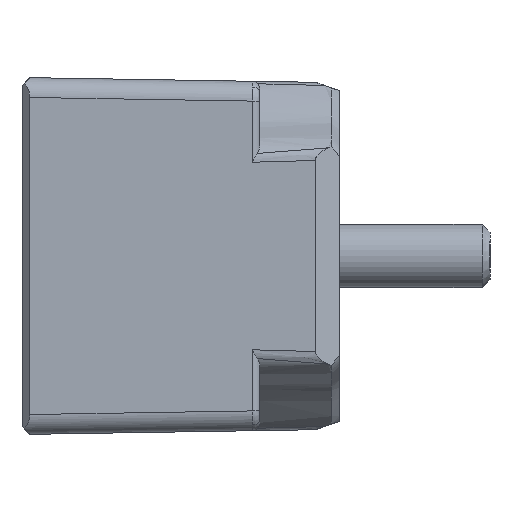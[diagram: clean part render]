
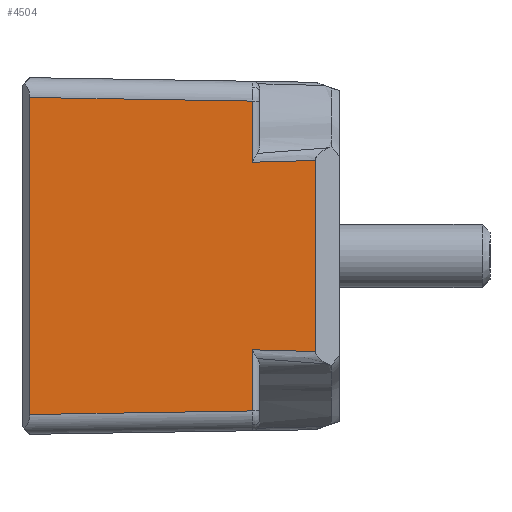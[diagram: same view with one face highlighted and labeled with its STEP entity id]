
A CAD part, left-side view. The second image highlights one B-rep face of the part: STEP entity #4504.
In plain terms, the highlighted planar face has unit normal (-1, -0.016, 0).
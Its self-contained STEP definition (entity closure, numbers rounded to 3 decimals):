
#189 = DIRECTION ( 'NONE',  ( -0.016, 1., 0.016 ) ) ;
#401 = CARTESIAN_POINT ( 'NONE',  ( -8.493, -0.1, -1.998 ) ) ;
#539 = CARTESIAN_POINT ( 'NONE',  ( -8.441, -3.302, -1.195 ) ) ;
#622 = CARTESIAN_POINT ( 'NONE',  ( -8.448, -2.902, 1.182 ) ) ;
#647 = CARTESIAN_POINT ( 'NONE',  ( -8.448, -2.902, -1.182 ) ) ;
#701 = CARTESIAN_POINT ( 'NONE',  ( -8.444, -3.169, -1.191 ) ) ;
#886 = ORIENTED_EDGE ( 'NONE', *, *, #1917, .T. ) ;
#990 = EDGE_CURVE ( 'NONE', #6883, #4766, #9644, .T. ) ;
#1015 = CARTESIAN_POINT ( 'NONE',  ( -8.448, -2.902, -1.182 ) ) ;
#1017 = VECTOR ( 'NONE', #8987, 1000. ) ;
#1172 = VECTOR ( 'NONE', #3954, 1000. ) ;
#1199 = EDGE_CURVE ( 'NONE', #4766, #1500, #3119, .T. ) ;
#1486 = EDGE_CURVE ( 'NONE', #8436, #5840, #6258, .T. ) ;
#1500 = VERTEX_POINT ( 'NONE', #4595 ) ;
#1817 = CARTESIAN_POINT ( 'NONE',  ( -8.435, -3.7, -1.204 ) ) ;
#1917 = EDGE_CURVE ( 'NONE', #3069, #4911, #2349, .T. ) ;
#2194 = VERTEX_POINT ( 'NONE', #622 ) ;
#2322 = VECTOR ( 'NONE', #7334, 1000. ) ;
#2349 = LINE ( 'NONE', #9001, #1172 ) ;
#2478 = EDGE_LOOP ( 'NONE', ( #2952, #8226, #8989, #6694, #8135, #886, #8292, #9587 ) ) ;
#2861 = DIRECTION ( 'NONE',  ( -1., -0.016, 0. ) ) ;
#2952 = ORIENTED_EDGE ( 'NONE', *, *, #1199, .T. ) ;
#3061 = CARTESIAN_POINT ( 'NONE',  ( -8.435, -3.7, 2.185 ) ) ;
#3069 = VERTEX_POINT ( 'NONE', #401 ) ;
#3119 = LINE ( 'NONE', #3061, #1017 ) ;
#3138 = CARTESIAN_POINT ( 'NONE',  ( -8.448, -2.902, -2.25 ) ) ;
#3382 = CARTESIAN_POINT ( 'NONE',  ( -8.441, -3.302, 1.195 ) ) ;
#3643 = CARTESIAN_POINT ( 'NONE',  ( -8.448, -2.902, -1.953 ) ) ;
#3954 = DIRECTION ( 'NONE',  ( 0.016, -1., 0.016 ) ) ;
#3985 = EDGE_CURVE ( 'NONE', #2194, #8436, #4789, .T. ) ;
#4006 = CARTESIAN_POINT ( 'NONE',  ( -8.435, -3.7, -1.204 ) ) ;
#4289 = LINE ( 'NONE', #6779, #5571 ) ;
#4504 = ADVANCED_FACE ( 'NONE', ( #8359 ), #9360, .T. ) ;
#4595 = CARTESIAN_POINT ( 'NONE',  ( -8.435, -3.7, 1.204 ) ) ;
#4607 = EDGE_CURVE ( 'NONE', #4911, #6883, #8063, .T. ) ;
#4766 = VERTEX_POINT ( 'NONE', #1817 ) ;
#4789 = LINE ( 'NONE', #6610, #2322 ) ;
#4911 = VERTEX_POINT ( 'NONE', #3643 ) ;
#4972 = CARTESIAN_POINT ( 'NONE',  ( -8.448, -2.902, 1.953 ) ) ;
#4981 = CARTESIAN_POINT ( 'NONE',  ( -8.437, -3.567, -1.202 ) ) ;
#5241 = CARTESIAN_POINT ( 'NONE',  ( -8.493, -0.1, 1.998 ) ) ;
#5571 = VECTOR ( 'NONE', #7658, 1000. ) ;
#5840 = VERTEX_POINT ( 'NONE', #5241 ) ;
#5843 = CARTESIAN_POINT ( 'NONE',  ( -8.448, -2.902, 1.182 ) ) ;
#5910 = EDGE_CURVE ( 'NONE', #5840, #3069, #4289, .T. ) ;
#6250 = DIRECTION ( 'NONE',  ( 0.016, -1., 0. ) ) ;
#6258 = LINE ( 'NONE', #8897, #9665 ) ;
#6599 = CARTESIAN_POINT ( 'NONE',  ( -8.435, -3.7, 1.204 ) ) ;
#6610 = CARTESIAN_POINT ( 'NONE',  ( -8.448, -2.902, -2.25 ) ) ;
#6694 = ORIENTED_EDGE ( 'NONE', *, *, #1486, .T. ) ;
#6779 = CARTESIAN_POINT ( 'NONE',  ( -8.493, -0.1, -2.25 ) ) ;
#6883 = VERTEX_POINT ( 'NONE', #1015 ) ;
#7334 = DIRECTION ( 'NONE',  ( 0., 0., 1. ) ) ;
#7484 = CARTESIAN_POINT ( 'NONE',  ( -8.437, -3.567, 1.202 ) ) ;
#7604 = VECTOR ( 'NONE', #10649, 1000. ) ;
#7658 = DIRECTION ( 'NONE',  ( 0., 0., -1. ) ) ;
#8063 = LINE ( 'NONE', #3138, #7604 ) ;
#8135 = ORIENTED_EDGE ( 'NONE', *, *, #5910, .T. ) ;
#8226 = ORIENTED_EDGE ( 'NONE', *, *, #8891, .T. ) ;
#8292 = ORIENTED_EDGE ( 'NONE', *, *, #4607, .T. ) ;
#8359 = FACE_OUTER_BOUND ( 'NONE', #2478, .T. ) ;
#8361 = CARTESIAN_POINT ( 'NONE',  ( -8.446, -3.035, 1.187 ) ) ;
#8436 = VERTEX_POINT ( 'NONE', #4972 ) ;
#8891 = EDGE_CURVE ( 'NONE', #1500, #2194, #8960, .T. ) ;
#8897 = CARTESIAN_POINT ( 'NONE',  ( -8.494, -0.069, 1.999 ) ) ;
#8941 = CARTESIAN_POINT ( 'NONE',  ( -8.439, -3.435, -1.198 ) ) ;
#8960 = B_SPLINE_CURVE_WITH_KNOTS ( 'NONE', 3,
 ( #6599, #7484, #9963, #3382, #10082, #8361, #5843 ),
 .UNSPECIFIED., .F., .F.,
 ( 4, 3, 4 ),
 ( 0., 0., 0.001 ),
 .UNSPECIFIED. ) ;
#8987 = DIRECTION ( 'NONE',  ( 0., 0., 1. ) ) ;
#8989 = ORIENTED_EDGE ( 'NONE', *, *, #3985, .T. ) ;
#9001 = CARTESIAN_POINT ( 'NONE',  ( -8.495, 0.004, -2. ) ) ;
#9104 = CARTESIAN_POINT ( 'NONE',  ( -8.446, -3.035, -1.187 ) ) ;
#9360 = PLANE ( 'NONE',  #9891 ) ;
#9587 = ORIENTED_EDGE ( 'NONE', *, *, #990, .T. ) ;
#9644 = B_SPLINE_CURVE_WITH_KNOTS ( 'NONE', 3,
 ( #647, #9104, #701, #539, #8941, #4981, #4006 ),
 .UNSPECIFIED., .F., .F.,
 ( 4, 3, 4 ),
 ( 0., 0., 0.001 ),
 .UNSPECIFIED. ) ;
#9665 = VECTOR ( 'NONE', #189, 1000. ) ;
#9891 = AXIS2_PLACEMENT_3D ( 'NONE', #10430, #2861, #6250 ) ;
#9963 = CARTESIAN_POINT ( 'NONE',  ( -8.439, -3.435, 1.198 ) ) ;
#10082 = CARTESIAN_POINT ( 'NONE',  ( -8.444, -3.169, 1.191 ) ) ;
#10430 = CARTESIAN_POINT ( 'NONE',  ( -8.495, 0., -2.25 ) ) ;
#10649 = DIRECTION ( 'NONE',  ( 0., 0., 1. ) ) ;
